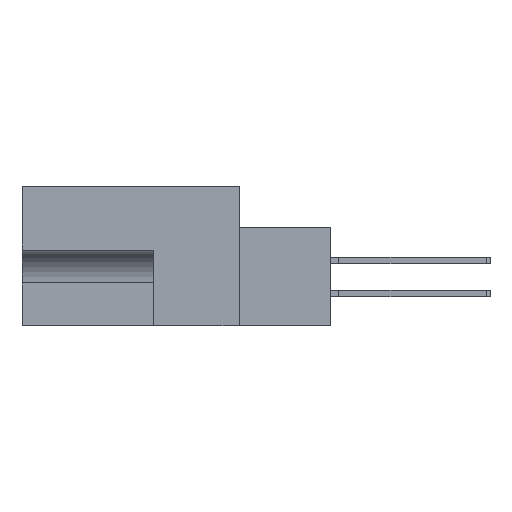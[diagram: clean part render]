
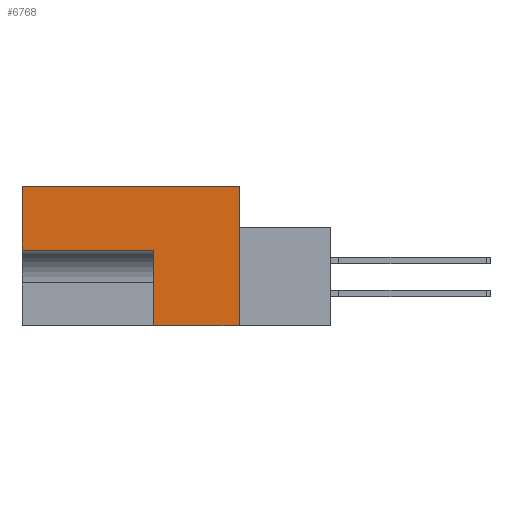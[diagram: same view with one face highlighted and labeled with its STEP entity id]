
A CAD part, left-side view. The second image highlights one B-rep face of the part: STEP entity #6768.
In plain terms, the highlighted planar face has unit normal (-1, 0, 0).
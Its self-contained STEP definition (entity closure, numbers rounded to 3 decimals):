
#173 = VECTOR ( 'NONE', #4059, 1000. ) ;
#410 = LINE ( 'NONE', #3594, #28547 ) ;
#639 = CARTESIAN_POINT ( 'NONE',  ( 0., 8.255, -13.487 ) ) ;
#2701 = PLANE ( 'NONE',  #31485 ) ;
#3594 = CARTESIAN_POINT ( 'NONE',  ( 0., 20.955, -13.487 ) ) ;
#4044 = LINE ( 'NONE', #30666, #17738 ) ;
#4059 = DIRECTION ( 'NONE',  ( 0., 1., 0. ) ) ;
#6454 = ORIENTED_EDGE ( 'NONE', *, *, #7387, .F. ) ;
#6482 = DIRECTION ( 'NONE',  ( 0., 0., -1. ) ) ;
#6563 = CARTESIAN_POINT ( 'NONE',  ( 0., -8.814, -13.487 ) ) ;
#6656 = LINE ( 'NONE', #14341, #13074 ) ;
#6768 = ADVANCED_FACE ( 'NONE', ( #22919 ), #2701, .F. ) ;
#7387 = EDGE_CURVE ( 'NONE', #25868, #30686, #6656, .T. ) ;
#7464 = LINE ( 'NONE', #14500, #27488 ) ;
#8991 = EDGE_CURVE ( 'NONE', #21239, #19079, #25785, .T. ) ;
#10768 = VERTEX_POINT ( 'NONE', #17824 ) ;
#13074 = VECTOR ( 'NONE', #33402, 1000. ) ;
#13528 = ORIENTED_EDGE ( 'NONE', *, *, #8991, .F. ) ;
#13570 = ORIENTED_EDGE ( 'NONE', *, *, #30198, .F. ) ;
#14341 = CARTESIAN_POINT ( 'NONE',  ( 0., 8.255, -6.172 ) ) ;
#14500 = CARTESIAN_POINT ( 'NONE',  ( 0., 0., 0. ) ) ;
#14662 = VECTOR ( 'NONE', #29203, 1000. ) ;
#15085 = LINE ( 'NONE', #26726, #14662 ) ;
#15137 = CARTESIAN_POINT ( 'NONE',  ( 0., 8.255, -6.172 ) ) ;
#17123 = DIRECTION ( 'NONE',  ( 0., -1., 0. ) ) ;
#17499 = ORIENTED_EDGE ( 'NONE', *, *, #33127, .F. ) ;
#17738 = VECTOR ( 'NONE', #17123, 1000. ) ;
#17824 = CARTESIAN_POINT ( 'NONE',  ( 0., 20.955, 0. ) ) ;
#17857 = ORIENTED_EDGE ( 'NONE', *, *, #24622, .F. ) ;
#18269 = ORIENTED_EDGE ( 'NONE', *, *, #29306, .F. ) ;
#19079 = VERTEX_POINT ( 'NONE', #639 ) ;
#19741 = DIRECTION ( 'NONE',  ( 0., 0., 1. ) ) ;
#21239 = VERTEX_POINT ( 'NONE', #32045 ) ;
#22267 = EDGE_LOOP ( 'NONE', ( #13528, #18269, #17857, #17499, #6454, #13570 ) ) ;
#22919 = FACE_OUTER_BOUND ( 'NONE', #22267, .T. ) ;
#24511 = CARTESIAN_POINT ( 'NONE',  ( 0., 0., 0. ) ) ;
#24622 = EDGE_CURVE ( 'NONE', #10768, #32452, #4044, .T. ) ;
#25785 = LINE ( 'NONE', #6563, #173 ) ;
#25868 = VERTEX_POINT ( 'NONE', #15137 ) ;
#26726 = CARTESIAN_POINT ( 'NONE',  ( 0., 8.255, -13.487 ) ) ;
#27485 = DIRECTION ( 'NONE',  ( 1., 0., 0. ) ) ;
#27488 = VECTOR ( 'NONE', #6482, 1000. ) ;
#28547 = VECTOR ( 'NONE', #19741, 1000. ) ;
#29043 = CARTESIAN_POINT ( 'NONE',  ( 0., 20.955, -6.172 ) ) ;
#29203 = DIRECTION ( 'NONE',  ( 0., 0., 1. ) ) ;
#29306 = EDGE_CURVE ( 'NONE', #32452, #21239, #7464, .T. ) ;
#30198 = EDGE_CURVE ( 'NONE', #19079, #25868, #15085, .T. ) ;
#30666 = CARTESIAN_POINT ( 'NONE',  ( 0., 11.506, 0. ) ) ;
#30686 = VERTEX_POINT ( 'NONE', #29043 ) ;
#31485 = AXIS2_PLACEMENT_3D ( 'NONE', #24511, #27485, #32845 ) ;
#32045 = CARTESIAN_POINT ( 'NONE',  ( 0., 0., -13.487 ) ) ;
#32452 = VERTEX_POINT ( 'NONE', #32976 ) ;
#32845 = DIRECTION ( 'NONE',  ( 0., 0., -1. ) ) ;
#32976 = CARTESIAN_POINT ( 'NONE',  ( 0., 0., 0. ) ) ;
#33127 = EDGE_CURVE ( 'NONE', #30686, #10768, #410, .T. ) ;
#33402 = DIRECTION ( 'NONE',  ( 0., 1., 0. ) ) ;
